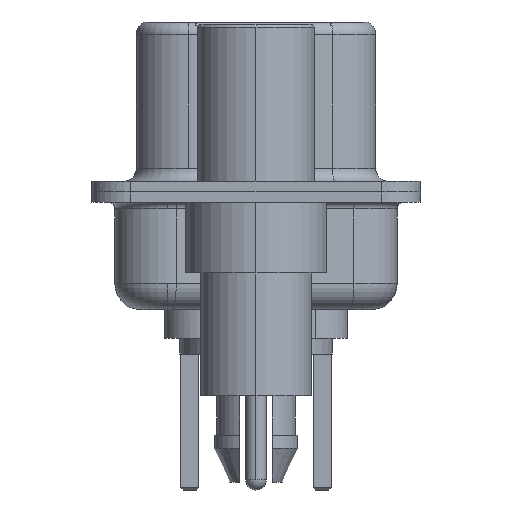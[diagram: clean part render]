
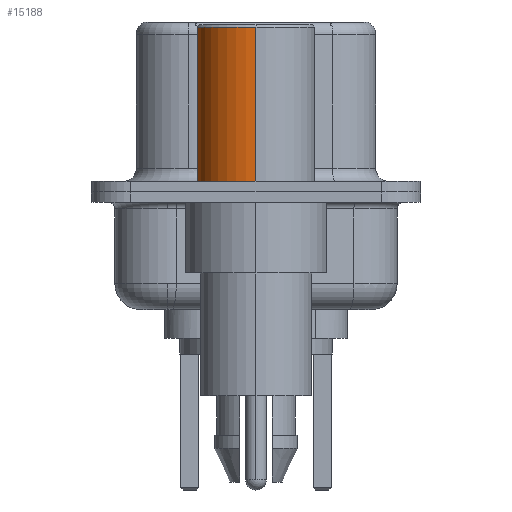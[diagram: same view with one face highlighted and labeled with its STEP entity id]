
A CAD part, left-side view. The second image highlights one B-rep face of the part: STEP entity #15188.
In plain terms, the highlighted cylindrical face has radius 2.25 mm (diameter 4.5 mm), a partial arc.
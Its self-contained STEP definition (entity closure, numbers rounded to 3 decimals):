
#443 = CARTESIAN_POINT ( 'NONE',  ( -2.25, 0., 6.3 ) ) ;
#819 = AXIS2_PLACEMENT_3D ( 'NONE', #15411, #7172, #7230 ) ;
#2241 = CIRCLE ( 'NONE', #4403, 2.25 ) ;
#2282 = DIRECTION ( 'NONE',  ( 1., 0., 0. ) ) ;
#2461 = DIRECTION ( 'NONE',  ( 0., 0., 1. ) ) ;
#3079 = VERTEX_POINT ( 'NONE', #16207 ) ;
#4349 = ORIENTED_EDGE ( 'NONE', *, *, #6780, .T. ) ;
#4403 = AXIS2_PLACEMENT_3D ( 'NONE', #9476, #12482, #2282 ) ;
#4758 = EDGE_CURVE ( 'NONE', #11444, #3079, #17200, .T. ) ;
#5274 = CARTESIAN_POINT ( 'NONE',  ( 2.25, 0., 0.4 ) ) ;
#5402 = VERTEX_POINT ( 'NONE', #443 ) ;
#6130 = VECTOR ( 'NONE', #2461, 1000. ) ;
#6780 = EDGE_CURVE ( 'NONE', #3079, #5402, #8664, .T. ) ;
#7172 = DIRECTION ( 'NONE',  ( 0., 0., 1. ) ) ;
#7230 = DIRECTION ( 'NONE',  ( 1., 0., 0. ) ) ;
#7482 = FACE_OUTER_BOUND ( 'NONE', #16805, .T. ) ;
#7677 = DIRECTION ( 'NONE',  ( 0., 0., 1. ) ) ;
#7858 = ORIENTED_EDGE ( 'NONE', *, *, #4758, .T. ) ;
#8557 = ORIENTED_EDGE ( 'NONE', *, *, #16210, .F. ) ;
#8589 = CARTESIAN_POINT ( 'NONE',  ( -2.25, 0., 0.581 ) ) ;
#8664 = LINE ( 'NONE', #8589, #6130 ) ;
#8793 = CARTESIAN_POINT ( 'NONE',  ( 2.25, 0., 6.3 ) ) ;
#9476 = CARTESIAN_POINT ( 'NONE',  ( 0., 0., 6.3 ) ) ;
#11444 = VERTEX_POINT ( 'NONE', #5274 ) ;
#11571 = DIRECTION ( 'NONE',  ( 0., 0., 1. ) ) ;
#12482 = DIRECTION ( 'NONE',  ( 0., 0., 1. ) ) ;
#12520 = ORIENTED_EDGE ( 'NONE', *, *, #15529, .F. ) ;
#13390 = CYLINDRICAL_SURFACE ( 'NONE', #819, 2.25 ) ;
#14328 = CARTESIAN_POINT ( 'NONE',  ( 0., 0., 0.4 ) ) ;
#14514 = DIRECTION ( 'NONE',  ( 1., 0., 0. ) ) ;
#15188 = ADVANCED_FACE ( 'NONE', ( #7482 ), #13390, .T. ) ;
#15323 = VERTEX_POINT ( 'NONE', #8793 ) ;
#15411 = CARTESIAN_POINT ( 'NONE',  ( 0., 0., 0.581 ) ) ;
#15529 = EDGE_CURVE ( 'NONE', #11444, #15323, #15578, .T. ) ;
#15578 = LINE ( 'NONE', #18016, #17184 ) ;
#16159 = AXIS2_PLACEMENT_3D ( 'NONE', #14328, #11571, #14514 ) ;
#16207 = CARTESIAN_POINT ( 'NONE',  ( -2.25, 0., 0.4 ) ) ;
#16210 = EDGE_CURVE ( 'NONE', #15323, #5402, #2241, .T. ) ;
#16805 = EDGE_LOOP ( 'NONE', ( #7858, #4349, #8557, #12520 ) ) ;
#17184 = VECTOR ( 'NONE', #7677, 1000. ) ;
#17200 = CIRCLE ( 'NONE', #16159, 2.25 ) ;
#18016 = CARTESIAN_POINT ( 'NONE',  ( 2.25, 0., 0.581 ) ) ;
